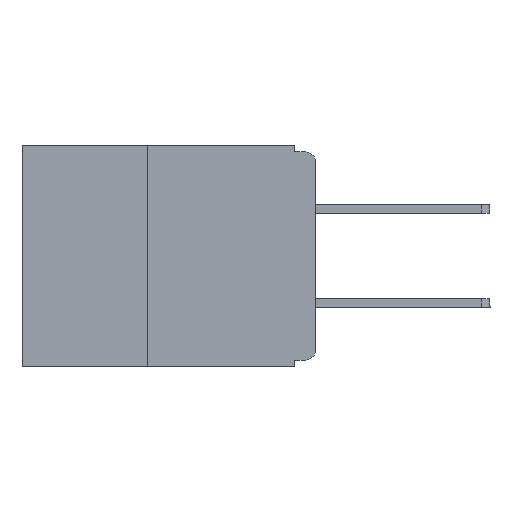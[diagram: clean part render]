
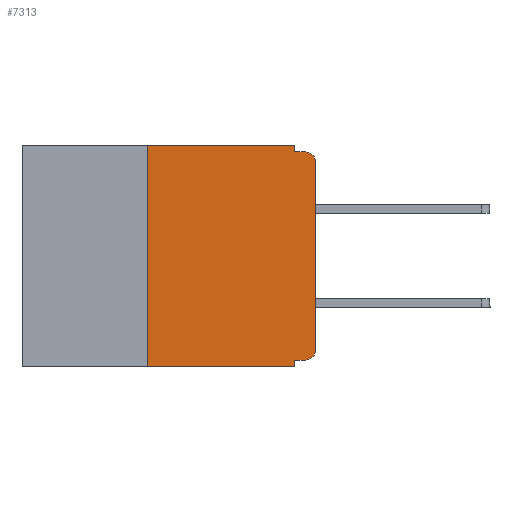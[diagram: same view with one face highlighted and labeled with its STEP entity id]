
A CAD part, left-side view. The second image highlights one B-rep face of the part: STEP entity #7313.
In plain terms, the highlighted planar face has unit normal (-1, 0, 0).
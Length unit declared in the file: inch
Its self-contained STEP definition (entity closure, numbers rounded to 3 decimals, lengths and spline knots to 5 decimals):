
#127 = VERTEX_POINT ( 'NONE', #4091 ) ;
#282 = CARTESIAN_POINT ( 'NONE',  ( 0., 0.25, -0.33 ) ) ;
#287 = DIRECTION ( 'NONE',  ( 0., 0., 1. ) ) ;
#517 = DIRECTION ( 'NONE',  ( 0., 0., -1. ) ) ;
#615 = VERTEX_POINT ( 'NONE', #11019 ) ;
#626 = DIRECTION ( 'NONE',  ( -1., 0., 0. ) ) ;
#887 = CARTESIAN_POINT ( 'NONE',  ( 0., 0.015, -0.305 ) ) ;
#1425 = CARTESIAN_POINT ( 'NONE',  ( 0., 0.437, 0. ) ) ;
#2374 = LINE ( 'NONE', #8786, #17888 ) ;
#2763 = EDGE_CURVE ( 'NONE', #10119, #6115, #4197, .T. ) ;
#2865 = LINE ( 'NONE', #8412, #13443 ) ;
#3083 = DIRECTION ( 'NONE',  ( 0., -1., 0. ) ) ;
#3138 = AXIS2_PLACEMENT_3D ( 'NONE', #14162, #4839, #15657 ) ;
#3219 = ORIENTED_EDGE ( 'NONE', *, *, #17346, .T. ) ;
#3463 = AXIS2_PLACEMENT_3D ( 'NONE', #887, #626, #517 ) ;
#3571 = EDGE_CURVE ( 'NONE', #4522, #14483, #10884, .T. ) ;
#3594 = CARTESIAN_POINT ( 'NONE',  ( 0., 0., -0.01 ) ) ;
#3612 = EDGE_CURVE ( 'NONE', #18952, #615, #2374, .T. ) ;
#3662 = CIRCLE ( 'NONE', #3463, 0.015 ) ;
#3816 = ORIENTED_EDGE ( 'NONE', *, *, #3571, .F. ) ;
#3864 = DIRECTION ( 'NONE',  ( 0., 0., -1. ) ) ;
#4026 = DIRECTION ( 'NONE',  ( 1., 0., 0. ) ) ;
#4048 = CARTESIAN_POINT ( 'NONE',  ( 0., 0.437, 0. ) ) ;
#4075 = PLANE ( 'NONE',  #11178 ) ;
#4091 = CARTESIAN_POINT ( 'NONE',  ( 0., 0.031, -0.33 ) ) ;
#4197 = LINE ( 'NONE', #15628, #19057 ) ;
#4522 = VERTEX_POINT ( 'NONE', #7484 ) ;
#4615 = CARTESIAN_POINT ( 'NONE',  ( 0., 0.031, 0. ) ) ;
#4839 = DIRECTION ( 'NONE',  ( -1., 0., 0. ) ) ;
#5343 = ORIENTED_EDGE ( 'NONE', *, *, #11139, .F. ) ;
#5531 = CARTESIAN_POINT ( 'NONE',  ( 0., 0., -0.32 ) ) ;
#6115 = VERTEX_POINT ( 'NONE', #8797 ) ;
#7313 = ADVANCED_FACE ( 'NONE', ( #17961 ), #4075, .F. ) ;
#7484 = CARTESIAN_POINT ( 'NONE',  ( 0., 0.031, -0.01 ) ) ;
#7625 = CARTESIAN_POINT ( 'NONE',  ( 0., 0.015, -0.32 ) ) ;
#8412 = CARTESIAN_POINT ( 'NONE',  ( 0., 0.031, -0.33 ) ) ;
#8786 = CARTESIAN_POINT ( 'NONE',  ( 0., 0., 0. ) ) ;
#8797 = CARTESIAN_POINT ( 'NONE',  ( 0., 0.25, 0. ) ) ;
#8852 = DIRECTION ( 'NONE',  ( 0., -1., 0. ) ) ;
#8881 = EDGE_CURVE ( 'NONE', #9843, #18952, #3662, .T. ) ;
#9190 = VECTOR ( 'NONE', #3083, 39.37008 ) ;
#9296 = DIRECTION ( 'NONE',  ( 0., 0., -1. ) ) ;
#9436 = EDGE_CURVE ( 'NONE', #6115, #10533, #13224, .T. ) ;
#9523 = DIRECTION ( 'NONE',  ( 0., -1., 0. ) ) ;
#9623 = EDGE_CURVE ( 'NONE', #15750, #127, #2865, .T. ) ;
#9763 = VECTOR ( 'NONE', #9523, 39.37008 ) ;
#9843 = VERTEX_POINT ( 'NONE', #7625 ) ;
#10054 = ORIENTED_EDGE ( 'NONE', *, *, #3612, .T. ) ;
#10119 = VERTEX_POINT ( 'NONE', #282 ) ;
#10533 = VERTEX_POINT ( 'NONE', #4615 ) ;
#10884 = LINE ( 'NONE', #3594, #14905 ) ;
#10893 = EDGE_CURVE ( 'NONE', #9843, #15750, #12908, .T. ) ;
#11019 = CARTESIAN_POINT ( 'NONE',  ( 0., 0., -0.025 ) ) ;
#11139 = EDGE_CURVE ( 'NONE', #10533, #4522, #16181, .T. ) ;
#11178 = AXIS2_PLACEMENT_3D ( 'NONE', #4048, #4026, #3864 ) ;
#12908 = LINE ( 'NONE', #5531, #19814 ) ;
#13179 = EDGE_CURVE ( 'NONE', #10119, #127, #14739, .T. ) ;
#13224 = LINE ( 'NONE', #1425, #9190 ) ;
#13443 = VECTOR ( 'NONE', #16015, 39.37008 ) ;
#13889 = CARTESIAN_POINT ( 'NONE',  ( 0., 0., -0.305 ) ) ;
#14010 = CARTESIAN_POINT ( 'NONE',  ( 0., 0.437, -0.33 ) ) ;
#14030 = ORIENTED_EDGE ( 'NONE', *, *, #8881, .T. ) ;
#14103 = CARTESIAN_POINT ( 'NONE',  ( 0., 0.015, -0.01 ) ) ;
#14162 = CARTESIAN_POINT ( 'NONE',  ( 0., 0.015, -0.025 ) ) ;
#14384 = ORIENTED_EDGE ( 'NONE', *, *, #10893, .F. ) ;
#14483 = VERTEX_POINT ( 'NONE', #14103 ) ;
#14632 = CARTESIAN_POINT ( 'NONE',  ( 0., 0.031, -0.32 ) ) ;
#14739 = LINE ( 'NONE', #14010, #9763 ) ;
#14819 = DIRECTION ( 'NONE',  ( 0., 1., 0. ) ) ;
#14905 = VECTOR ( 'NONE', #8852, 39.37008 ) ;
#15424 = ORIENTED_EDGE ( 'NONE', *, *, #9623, .F. ) ;
#15628 = CARTESIAN_POINT ( 'NONE',  ( 0., 0.25, -0.33 ) ) ;
#15657 = DIRECTION ( 'NONE',  ( 0., 0., -1. ) ) ;
#15700 = VECTOR ( 'NONE', #9296, 39.37008 ) ;
#15750 = VERTEX_POINT ( 'NONE', #14632 ) ;
#16015 = DIRECTION ( 'NONE',  ( 0., 0., -1. ) ) ;
#16090 = ORIENTED_EDGE ( 'NONE', *, *, #13179, .T. ) ;
#16181 = LINE ( 'NONE', #19777, #15700 ) ;
#17346 = EDGE_CURVE ( 'NONE', #615, #14483, #19769, .T. ) ;
#17409 = ORIENTED_EDGE ( 'NONE', *, *, #2763, .F. ) ;
#17864 = EDGE_LOOP ( 'NONE', ( #10054, #3219, #3816, #5343, #19844, #17409, #16090, #15424, #14384, #14030 ) ) ;
#17888 = VECTOR ( 'NONE', #287, 39.37008 ) ;
#17961 = FACE_OUTER_BOUND ( 'NONE', #17864, .T. ) ;
#18763 = DIRECTION ( 'NONE',  ( 0., 0., 1. ) ) ;
#18952 = VERTEX_POINT ( 'NONE', #13889 ) ;
#19057 = VECTOR ( 'NONE', #18763, 39.37008 ) ;
#19769 = CIRCLE ( 'NONE', #3138, 0.015 ) ;
#19777 = CARTESIAN_POINT ( 'NONE',  ( 0., 0.031, 0. ) ) ;
#19814 = VECTOR ( 'NONE', #14819, 39.37008 ) ;
#19844 = ORIENTED_EDGE ( 'NONE', *, *, #9436, .F. ) ;
